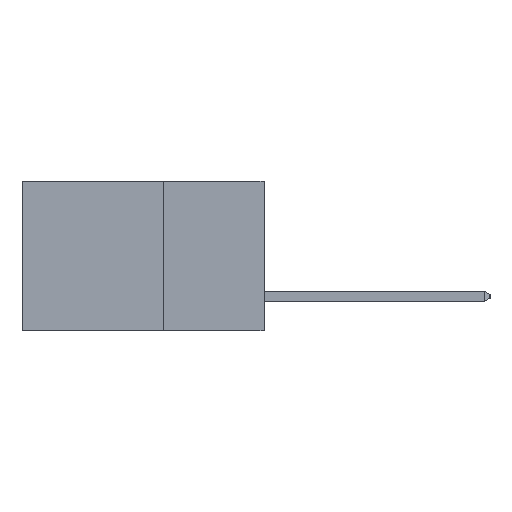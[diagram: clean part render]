
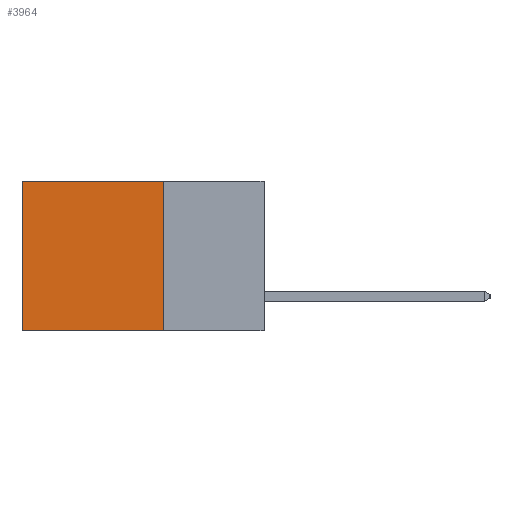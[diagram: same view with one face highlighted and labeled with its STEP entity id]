
A CAD part, left-side view. The second image highlights one B-rep face of the part: STEP entity #3964.
In plain terms, the highlighted planar face has unit normal (-1, 0, 0).
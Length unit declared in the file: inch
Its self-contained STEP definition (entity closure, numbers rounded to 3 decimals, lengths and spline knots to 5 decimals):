
#6 = EDGE_CURVE ( 'NONE', #15390, #10049, #4880, .T. ) ;
#294 = LINE ( 'NONE', #3000, #10655 ) ;
#1091 = VECTOR ( 'NONE', #14530, 39.37008 ) ;
#1553 = DIRECTION ( 'NONE',  ( 0., 0., -1. ) ) ;
#1712 = CARTESIAN_POINT ( 'NONE',  ( 0.2615, 0.25, 0. ) ) ;
#1882 = EDGE_LOOP ( 'NONE', ( #3681, #15222, #12822, #11546 ) ) ;
#3000 = CARTESIAN_POINT ( 'NONE',  ( 0.2615, 0.6, -0.37 ) ) ;
#3043 = PLANE ( 'NONE',  #9472 ) ;
#3539 = LINE ( 'NONE', #10239, #10927 ) ;
#3681 = ORIENTED_EDGE ( 'NONE', *, *, #16394, .T. ) ;
#3964 = ADVANCED_FACE ( 'NONE', ( #7993 ), #3043, .F. ) ;
#4130 = CARTESIAN_POINT ( 'NONE',  ( 0.2615, 0.25, 0. ) ) ;
#4328 = LINE ( 'NONE', #5332, #1091 ) ;
#4880 = LINE ( 'NONE', #1712, #8387 ) ;
#5306 = EDGE_CURVE ( 'NONE', #11763, #8209, #3539, .T. ) ;
#5332 = CARTESIAN_POINT ( 'NONE',  ( 0.2615, 0.25, -0.37 ) ) ;
#5653 = DIRECTION ( 'NONE',  ( 1., 0., 0. ) ) ;
#7993 = FACE_OUTER_BOUND ( 'NONE', #1882, .T. ) ;
#8209 = VERTEX_POINT ( 'NONE', #16999 ) ;
#8249 = CARTESIAN_POINT ( 'NONE',  ( 0.2615, 0.25, -0.37 ) ) ;
#8387 = VECTOR ( 'NONE', #8767, 39.37008 ) ;
#8767 = DIRECTION ( 'NONE',  ( 0., 1., 0. ) ) ;
#9472 = AXIS2_PLACEMENT_3D ( 'NONE', #8249, #5653, #14852 ) ;
#10049 = VERTEX_POINT ( 'NONE', #10172 ) ;
#10172 = CARTESIAN_POINT ( 'NONE',  ( 0.2615, 0.6, 0. ) ) ;
#10239 = CARTESIAN_POINT ( 'NONE',  ( 0.2615, 0.25, -0.37 ) ) ;
#10655 = VECTOR ( 'NONE', #1553, 39.37008 ) ;
#10927 = VECTOR ( 'NONE', #14073, 39.37008 ) ;
#11546 = ORIENTED_EDGE ( 'NONE', *, *, #6, .T. ) ;
#11763 = VERTEX_POINT ( 'NONE', #13512 ) ;
#12822 = ORIENTED_EDGE ( 'NONE', *, *, #13099, .F. ) ;
#13099 = EDGE_CURVE ( 'NONE', #15390, #11763, #4328, .T. ) ;
#13512 = CARTESIAN_POINT ( 'NONE',  ( 0.2615, 0.25, -0.37 ) ) ;
#14073 = DIRECTION ( 'NONE',  ( 0., 1., 0. ) ) ;
#14530 = DIRECTION ( 'NONE',  ( 0., 0., -1. ) ) ;
#14852 = DIRECTION ( 'NONE',  ( 0., 0., -1. ) ) ;
#15222 = ORIENTED_EDGE ( 'NONE', *, *, #5306, .F. ) ;
#15390 = VERTEX_POINT ( 'NONE', #4130 ) ;
#16394 = EDGE_CURVE ( 'NONE', #10049, #8209, #294, .T. ) ;
#16999 = CARTESIAN_POINT ( 'NONE',  ( 0.2615, 0.6, -0.37 ) ) ;
